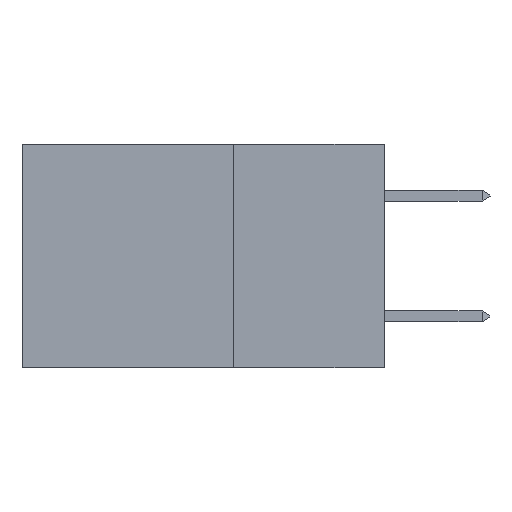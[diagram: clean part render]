
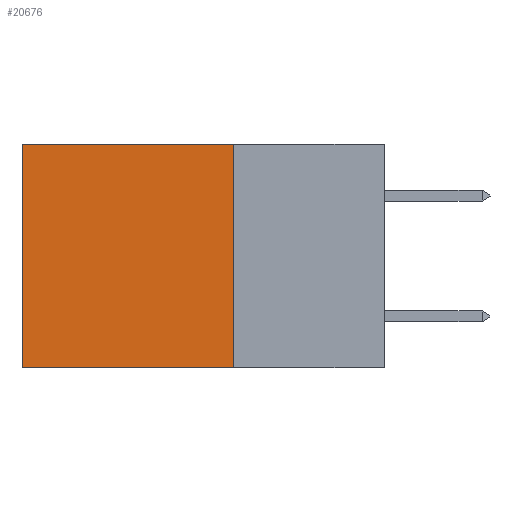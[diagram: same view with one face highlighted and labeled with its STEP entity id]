
A CAD part, left-side view. The second image highlights one B-rep face of the part: STEP entity #20676.
In plain terms, the highlighted planar face has unit normal (-1, 0, 0).
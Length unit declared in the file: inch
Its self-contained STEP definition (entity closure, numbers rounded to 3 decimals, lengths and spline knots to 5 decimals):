
#431 = EDGE_CURVE ( 'NONE', #4786, #41735, #977, .T. ) ;
#977 = LINE ( 'NONE', #20778, #8964 ) ;
#2624 = EDGE_CURVE ( 'NONE', #4786, #15041, #3131, .T. ) ;
#3131 = LINE ( 'NONE', #40492, #14776 ) ;
#3274 = DIRECTION ( 'NONE',  ( 0., 0., -1. ) ) ;
#4291 = ORIENTED_EDGE ( 'NONE', *, *, #2624, .T. ) ;
#4786 = VERTEX_POINT ( 'NONE', #32391 ) ;
#6388 = CARTESIAN_POINT ( 'NONE',  ( 0.2875, 0.6, 0. ) ) ;
#8964 = VECTOR ( 'NONE', #20554, 39.37008 ) ;
#9078 = ORIENTED_EDGE ( 'NONE', *, *, #19429, .T. ) ;
#9413 = VECTOR ( 'NONE', #3274, 39.37008 ) ;
#12138 = VERTEX_POINT ( 'NONE', #35361 ) ;
#14776 = VECTOR ( 'NONE', #16671, 39.37008 ) ;
#15041 = VERTEX_POINT ( 'NONE', #24224 ) ;
#15433 = EDGE_CURVE ( 'NONE', #41735, #12138, #36471, .T. ) ;
#16671 = DIRECTION ( 'NONE',  ( 0., 1., 0. ) ) ;
#16960 = CARTESIAN_POINT ( 'NONE',  ( 0.2875, 0.25, -0.37 ) ) ;
#19429 = EDGE_CURVE ( 'NONE', #15041, #12138, #30606, .T. ) ;
#20554 = DIRECTION ( 'NONE',  ( 0., 0., -1. ) ) ;
#20676 = ADVANCED_FACE ( 'NONE', ( #36201 ), #22634, .F. ) ;
#20778 = CARTESIAN_POINT ( 'NONE',  ( 0.2875, 0.25, 0. ) ) ;
#22634 = PLANE ( 'NONE',  #30079 ) ;
#22857 = DIRECTION ( 'NONE',  ( 0., 0., -1. ) ) ;
#22903 = DIRECTION ( 'NONE',  ( 0., 1., 0. ) ) ;
#23089 = ORIENTED_EDGE ( 'NONE', *, *, #15433, .F. ) ;
#24224 = CARTESIAN_POINT ( 'NONE',  ( 0.2875, 0.6, 0. ) ) ;
#24358 = EDGE_LOOP ( 'NONE', ( #9078, #23089, #38914, #4291 ) ) ;
#26203 = DIRECTION ( 'NONE',  ( 1., 0., 0. ) ) ;
#29538 = CARTESIAN_POINT ( 'NONE',  ( 0.2875, 0.25, 0. ) ) ;
#30079 = AXIS2_PLACEMENT_3D ( 'NONE', #29538, #26203, #22857 ) ;
#30606 = LINE ( 'NONE', #6388, #9413 ) ;
#32391 = CARTESIAN_POINT ( 'NONE',  ( 0.2875, 0.25, 0. ) ) ;
#32469 = CARTESIAN_POINT ( 'NONE',  ( 0.2875, 0.25, -0.37 ) ) ;
#35361 = CARTESIAN_POINT ( 'NONE',  ( 0.2875, 0.6, -0.37 ) ) ;
#36201 = FACE_OUTER_BOUND ( 'NONE', #24358, .T. ) ;
#36471 = LINE ( 'NONE', #32469, #42634 ) ;
#38914 = ORIENTED_EDGE ( 'NONE', *, *, #431, .F. ) ;
#40492 = CARTESIAN_POINT ( 'NONE',  ( 0.2875, 0.25, 0. ) ) ;
#41735 = VERTEX_POINT ( 'NONE', #16960 ) ;
#42634 = VECTOR ( 'NONE', #22903, 39.37008 ) ;
